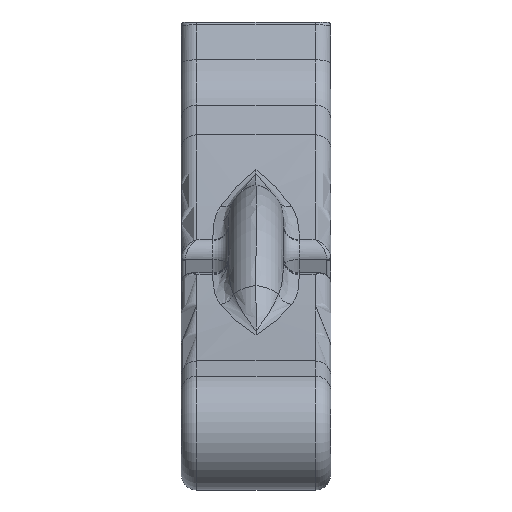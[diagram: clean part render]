
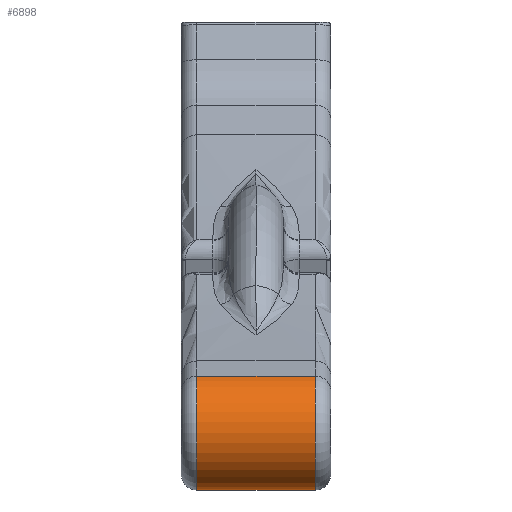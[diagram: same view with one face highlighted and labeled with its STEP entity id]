
A CAD part, front view. The second image highlights one B-rep face of the part: STEP entity #6898.
In plain terms, the highlighted cylindrical face has radius 3.75 mm (diameter 7.5 mm), a partial arc.
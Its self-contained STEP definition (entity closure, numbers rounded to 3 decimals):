
#6 = CARTESIAN_POINT ( 'NONE',  ( 8.5, -1.393, 3.482 ) ) ;
#267 = DIRECTION ( 'NONE',  ( -1., 0., 0. ) ) ;
#654 = DIRECTION ( 'NONE',  ( 1., 0., 0. ) ) ;
#697 = ORIENTED_EDGE ( 'NONE', *, *, #2355, .T. ) ;
#1498 = FACE_OUTER_BOUND ( 'NONE', #4341, .T. ) ;
#1523 = VECTOR ( 'NONE', #5515, 1000. ) ;
#1696 = DIRECTION ( 'NONE',  ( -1., 0., 0. ) ) ;
#2060 = ORIENTED_EDGE ( 'NONE', *, *, #3979, .T. ) ;
#2072 = ORIENTED_EDGE ( 'NONE', *, *, #2172, .F. ) ;
#2109 = AXIS2_PLACEMENT_3D ( 'NONE', #2722, #6764, #3310 ) ;
#2172 = EDGE_CURVE ( 'NONE', #5693, #2947, #4369, .T. ) ;
#2289 = DIRECTION ( 'NONE',  ( 0., 0., 1. ) ) ;
#2341 = EDGE_CURVE ( 'NONE', #7225, #7293, #3110, .T. ) ;
#2355 = EDGE_CURVE ( 'NONE', #7225, #2947, #4628, .T. ) ;
#2403 = CARTESIAN_POINT ( 'NONE',  ( 9.5, -1.393, 3.482 ) ) ;
#2520 = CYLINDRICAL_SURFACE ( 'NONE', #6726, 3.75 ) ;
#2635 = VECTOR ( 'NONE', #654, 1000. ) ;
#2722 = CARTESIAN_POINT ( 'NONE',  ( 1., 0., 0. ) ) ;
#2947 = VERTEX_POINT ( 'NONE', #6 ) ;
#3110 = LINE ( 'NONE', #4926, #1523 ) ;
#3310 = DIRECTION ( 'NONE',  ( 0., 0., 1. ) ) ;
#3374 = CARTESIAN_POINT ( 'NONE',  ( 8.5, 1.393, -3.482 ) ) ;
#3775 = CARTESIAN_POINT ( 'NONE',  ( 8.5, 0., 0. ) ) ;
#3914 = AXIS2_PLACEMENT_3D ( 'NONE', #3775, #267, #4357 ) ;
#3979 = EDGE_CURVE ( 'NONE', #5693, #7293, #7031, .T. ) ;
#4341 = EDGE_LOOP ( 'NONE', ( #6111, #697, #2072, #2060 ) ) ;
#4357 = DIRECTION ( 'NONE',  ( 0., 0., 1. ) ) ;
#4369 = LINE ( 'NONE', #2403, #2635 ) ;
#4611 = CARTESIAN_POINT ( 'NONE',  ( 1., 1.393, -3.482 ) ) ;
#4628 = CIRCLE ( 'NONE', #3914, 3.75 ) ;
#4643 = CARTESIAN_POINT ( 'NONE',  ( 1., -1.393, 3.482 ) ) ;
#4926 = CARTESIAN_POINT ( 'NONE',  ( 9.5, 1.393, -3.482 ) ) ;
#5515 = DIRECTION ( 'NONE',  ( -1., 0., 0. ) ) ;
#5693 = VERTEX_POINT ( 'NONE', #4643 ) ;
#5780 = CARTESIAN_POINT ( 'NONE',  ( 9.5, 0., 0. ) ) ;
#6111 = ORIENTED_EDGE ( 'NONE', *, *, #2341, .F. ) ;
#6726 = AXIS2_PLACEMENT_3D ( 'NONE', #5780, #1696, #2289 ) ;
#6764 = DIRECTION ( 'NONE',  ( 1., 0., 0. ) ) ;
#6898 = ADVANCED_FACE ( 'NONE', ( #1498 ), #2520, .T. ) ;
#7031 = CIRCLE ( 'NONE', #2109, 3.75 ) ;
#7225 = VERTEX_POINT ( 'NONE', #3374 ) ;
#7293 = VERTEX_POINT ( 'NONE', #4611 ) ;
